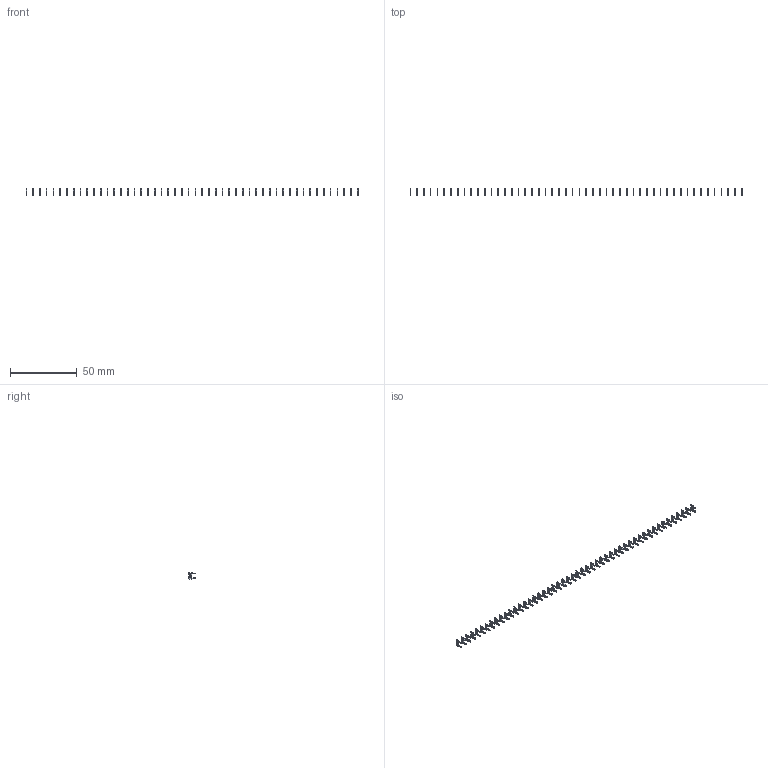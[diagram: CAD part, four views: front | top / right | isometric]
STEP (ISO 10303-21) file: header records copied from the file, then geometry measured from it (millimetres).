
FILE_DESCRIPTION (( 'STEP AP203' ), '1' );
FILE_NAME ('105-050-208-200.STEP', '2020-04-08T00:27:32', ( '' ), ( '' ), 'SwSTEP 2.0', 'SolidWorks 2016', '' );
FILE_SCHEMA (( 'CONFIG_CONTROL_DESIGN' ));
Length unit declared in the file: inch
Products named in the file (2): 105-050-208-200; 100-290-001_100-290-208
Assembly tree (50 placements, depth 2):
  105-050-208-200
    100-290-001_100-290-208  x50
Bounding box: 249.43 x 4.83 x 5.17 mm (x, y, z)
Volume: 344 mm3; surface area: 2124.8 mm2
Topology: 50 solids, 50 shells, 1250 faces, 3450 edges, 2300 vertices
Faces by surface type: plane 1100, cylinder 150
Entity records: 2557 total; most frequent: DIRECTION 231, CARTESIAN_POINT 193, ORIENTED_EDGE 138, COORDINATED_UNIVERSAL_TIME_OFFSET 110, CALENDAR_DATE 110, DATE_AND_TIME 110, LOCAL_TIME 110, AXIS2_PLACEMENT_3D 84
